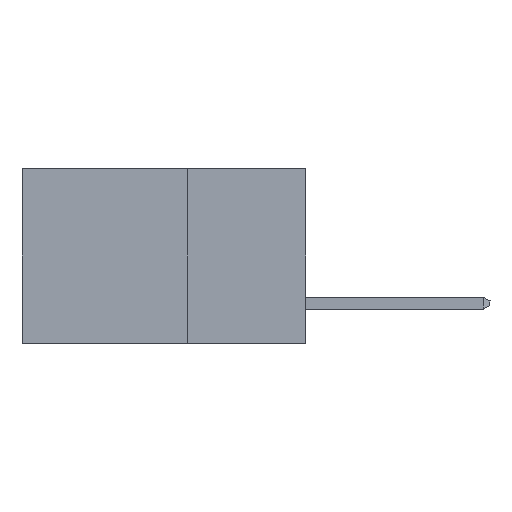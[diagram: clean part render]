
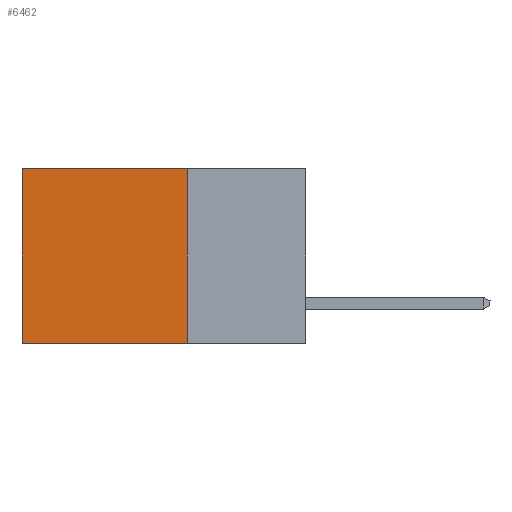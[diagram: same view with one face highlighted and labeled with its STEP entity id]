
A CAD part, left-side view. The second image highlights one B-rep face of the part: STEP entity #6462.
In plain terms, the highlighted planar face has unit normal (-1, 0, 0).
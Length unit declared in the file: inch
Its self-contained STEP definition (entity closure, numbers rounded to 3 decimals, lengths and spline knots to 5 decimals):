
#686 = PLANE ( 'NONE',  #2984 ) ;
#1031 = VERTEX_POINT ( 'NONE', #11241 ) ;
#1147 = LINE ( 'NONE', #13761, #10483 ) ;
#1265 = VECTOR ( 'NONE', #7074, 39.37008 ) ;
#2425 = ORIENTED_EDGE ( 'NONE', *, *, #9973, .F. ) ;
#2463 = DIRECTION ( 'NONE',  ( 0., 0., -1. ) ) ;
#2984 = AXIS2_PLACEMENT_3D ( 'NONE', #13882, #9947, #15146 ) ;
#3227 = FACE_OUTER_BOUND ( 'NONE', #9468, .T. ) ;
#3401 = ORIENTED_EDGE ( 'NONE', *, *, #11081, .F. ) ;
#4437 = ORIENTED_EDGE ( 'NONE', *, *, #10971, .T. ) ;
#4912 = CARTESIAN_POINT ( 'NONE',  ( 0.298, 0.25, 0. ) ) ;
#5216 = CARTESIAN_POINT ( 'NONE',  ( 0.298, 0.25, 0. ) ) ;
#6462 = ADVANCED_FACE ( 'NONE', ( #3227 ), #686, .F. ) ;
#6552 = DIRECTION ( 'NONE',  ( 0., 1., 0. ) ) ;
#6743 = VERTEX_POINT ( 'NONE', #4912 ) ;
#7014 = ORIENTED_EDGE ( 'NONE', *, *, #15900, .T. ) ;
#7074 = DIRECTION ( 'NONE',  ( 0., 1., 0. ) ) ;
#9468 = EDGE_LOOP ( 'NONE', ( #7014, #2425, #3401, #4437 ) ) ;
#9947 = DIRECTION ( 'NONE',  ( 1., 0., 0. ) ) ;
#9973 = EDGE_CURVE ( 'NONE', #1031, #15290, #13242, .T. ) ;
#10483 = VECTOR ( 'NONE', #11315, 39.37008 ) ;
#10542 = VECTOR ( 'NONE', #2463, 39.37008 ) ;
#10940 = CARTESIAN_POINT ( 'NONE',  ( 0.298, 0.25, -0.37 ) ) ;
#10971 = EDGE_CURVE ( 'NONE', #6743, #12725, #14624, .T. ) ;
#11071 = CARTESIAN_POINT ( 'NONE',  ( 0.298, 0.6, -0.37 ) ) ;
#11081 = EDGE_CURVE ( 'NONE', #6743, #1031, #14007, .T. ) ;
#11241 = CARTESIAN_POINT ( 'NONE',  ( 0.298, 0.25, -0.37 ) ) ;
#11315 = DIRECTION ( 'NONE',  ( 0., 0., -1. ) ) ;
#12725 = VERTEX_POINT ( 'NONE', #14969 ) ;
#13198 = VECTOR ( 'NONE', #6552, 39.37008 ) ;
#13242 = LINE ( 'NONE', #10940, #1265 ) ;
#13761 = CARTESIAN_POINT ( 'NONE',  ( 0.298, 0.6, 0. ) ) ;
#13882 = CARTESIAN_POINT ( 'NONE',  ( 0.298, 0.25, 0. ) ) ;
#14007 = LINE ( 'NONE', #17092, #10542 ) ;
#14624 = LINE ( 'NONE', #5216, #13198 ) ;
#14969 = CARTESIAN_POINT ( 'NONE',  ( 0.298, 0.6, 0. ) ) ;
#15146 = DIRECTION ( 'NONE',  ( 0., 0., -1. ) ) ;
#15290 = VERTEX_POINT ( 'NONE', #11071 ) ;
#15900 = EDGE_CURVE ( 'NONE', #12725, #15290, #1147, .T. ) ;
#17092 = CARTESIAN_POINT ( 'NONE',  ( 0.298, 0.25, 0. ) ) ;
